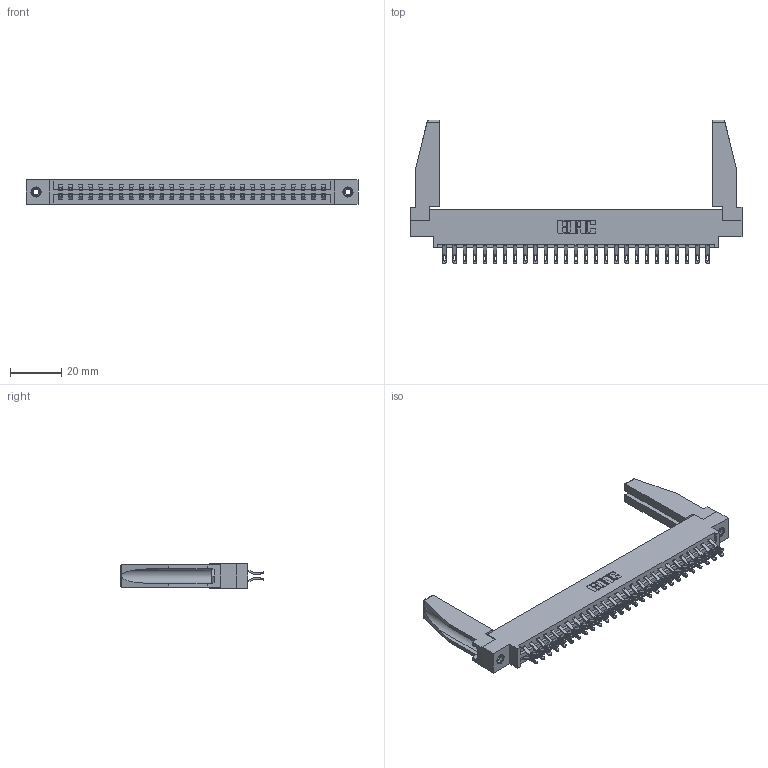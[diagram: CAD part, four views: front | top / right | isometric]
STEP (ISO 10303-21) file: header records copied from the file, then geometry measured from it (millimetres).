
FILE_DESCRIPTION (( 'STEP AP203' ), '1' );
FILE_NAME ('387-054-555-878.STEP', '2019-10-19T05:32:09', ( '' ), ( '' ), 'SwSTEP 2.0', 'SolidWorks 2016', '' );
FILE_SCHEMA (( 'CONFIG_CONTROL_DESIGN' ));
Length unit declared in the file: inch
Products named in the file (5): 345-250-001_345-250-001-102; 307-220-078; 337 Part_0.170 Offset - 0.156 Dia-TI; 345-292-001_555 Tail; 387-054-555-878
Assembly tree (59 placements, depth 2):
  387-054-555-878
    337 Part_0.170 Offset - 0.156 Dia-TI
    345-292-001_555 Tail  x54
    345-250-001_345-250-001-102  x2
    307-220-078  x2
Bounding box: 130 x 56.27 x 9.4 mm (x, y, z)
Volume: 17532.9 mm3; surface area: 19689.4 mm2
Topology: 59 solids, 59 shells, 3488 faces, 10859 edges, 7230 vertices
Faces by surface type: plane 2102, cylinder 1370, cone 12, torus 4
Entity records: 25772 total; most frequent: CARTESIAN_POINT 4390, ORIENTED_EDGE 4252, DIRECTION 3738, EDGE_CURVE 2126, LINE 1940, VECTOR 1940, VERTEX_POINT 1412, AXIS2_PLACEMENT_3D 899
